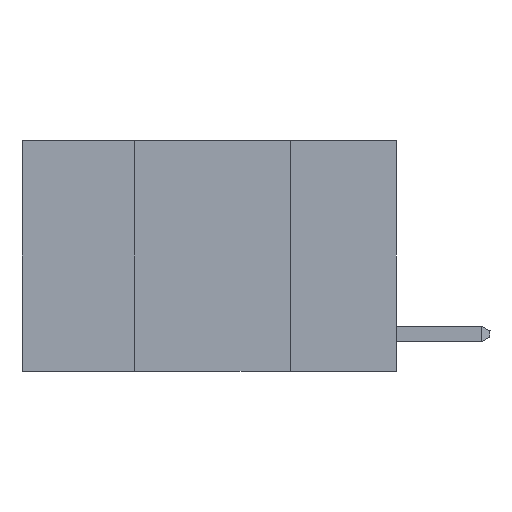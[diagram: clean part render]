
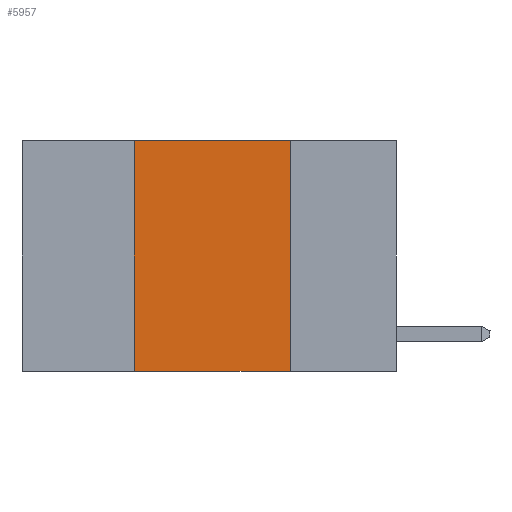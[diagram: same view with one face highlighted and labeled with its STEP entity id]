
A CAD part, left-side view. The second image highlights one B-rep face of the part: STEP entity #5957.
In plain terms, the highlighted planar face has unit normal (-1, 0, 0).
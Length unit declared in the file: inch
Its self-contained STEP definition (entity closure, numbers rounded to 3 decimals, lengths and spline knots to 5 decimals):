
#44 = CARTESIAN_POINT ( 'NONE',  ( 0., 0.6, -0.37 ) ) ;
#304 = EDGE_CURVE ( 'NONE', #16531, #3632, #2055, .T. ) ;
#458 = EDGE_CURVE ( 'NONE', #5617, #17189, #6254, .T. ) ;
#552 = EDGE_CURVE ( 'NONE', #5617, #3632, #11256, .T. ) ;
#933 = DIRECTION ( 'NONE',  ( 1., 0., 0. ) ) ;
#2055 = LINE ( 'NONE', #16790, #9014 ) ;
#2288 = CARTESIAN_POINT ( 'NONE',  ( 0., 0.17, -0.37 ) ) ;
#2448 = VECTOR ( 'NONE', #3158, 39.37008 ) ;
#3079 = ORIENTED_EDGE ( 'NONE', *, *, #304, .F. ) ;
#3158 = DIRECTION ( 'NONE',  ( 0., -1., 0. ) ) ;
#3461 = ORIENTED_EDGE ( 'NONE', *, *, #7986, .F. ) ;
#3498 = ORIENTED_EDGE ( 'NONE', *, *, #458, .F. ) ;
#3632 = VERTEX_POINT ( 'NONE', #2288 ) ;
#3708 = ORIENTED_EDGE ( 'NONE', *, *, #552, .T. ) ;
#4416 = FACE_OUTER_BOUND ( 'NONE', #15685, .T. ) ;
#5617 = VERTEX_POINT ( 'NONE', #6170 ) ;
#5957 = ADVANCED_FACE ( 'NONE', ( #4416 ), #9809, .F. ) ;
#6170 = CARTESIAN_POINT ( 'NONE',  ( 0., 0.42, -0.37 ) ) ;
#6254 = LINE ( 'NONE', #13028, #10586 ) ;
#6429 = LINE ( 'NONE', #11897, #2448 ) ;
#7986 = EDGE_CURVE ( 'NONE', #17189, #16531, #6429, .T. ) ;
#9014 = VECTOR ( 'NONE', #14084, 39.37008 ) ;
#9809 = PLANE ( 'NONE',  #10954 ) ;
#10586 = VECTOR ( 'NONE', #17129, 39.37008 ) ;
#10954 = AXIS2_PLACEMENT_3D ( 'NONE', #15411, #933, #11250 ) ;
#11250 = DIRECTION ( 'NONE',  ( 0., 0., -1. ) ) ;
#11256 = LINE ( 'NONE', #44, #14992 ) ;
#11897 = CARTESIAN_POINT ( 'NONE',  ( 0., 0.6, 0. ) ) ;
#12649 = CARTESIAN_POINT ( 'NONE',  ( 0., 0.17, 0. ) ) ;
#13028 = CARTESIAN_POINT ( 'NONE',  ( 0., 0.42, 0. ) ) ;
#14084 = DIRECTION ( 'NONE',  ( 0., 0., -1. ) ) ;
#14992 = VECTOR ( 'NONE', #15999, 39.37008 ) ;
#15411 = CARTESIAN_POINT ( 'NONE',  ( 0., 0.6, 0. ) ) ;
#15685 = EDGE_LOOP ( 'NONE', ( #3079, #3461, #3498, #3708 ) ) ;
#15999 = DIRECTION ( 'NONE',  ( 0., -1., 0. ) ) ;
#16531 = VERTEX_POINT ( 'NONE', #12649 ) ;
#16790 = CARTESIAN_POINT ( 'NONE',  ( 0., 0.17, 0. ) ) ;
#17129 = DIRECTION ( 'NONE',  ( 0., 0., 1. ) ) ;
#17189 = VERTEX_POINT ( 'NONE', #17771 ) ;
#17771 = CARTESIAN_POINT ( 'NONE',  ( 0., 0.42, 0. ) ) ;
